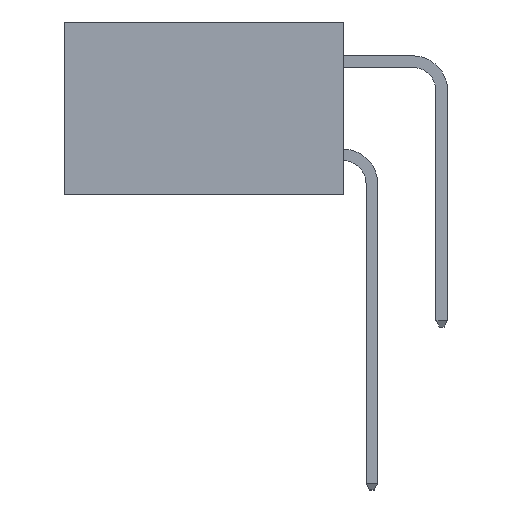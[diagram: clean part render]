
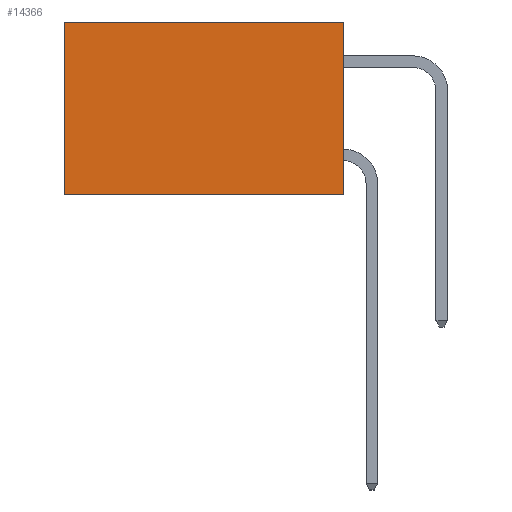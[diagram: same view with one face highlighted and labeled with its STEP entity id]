
A CAD part, left-side view. The second image highlights one B-rep face of the part: STEP entity #14366.
In plain terms, the highlighted planar face has unit normal (-1, 0, 0).
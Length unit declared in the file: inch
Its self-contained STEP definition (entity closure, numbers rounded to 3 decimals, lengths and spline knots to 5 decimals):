
#51 = VERTEX_POINT ( 'NONE', #115 ) ;
#115 = CARTESIAN_POINT ( 'NONE',  ( 0.2615, 0.6, 0. ) ) ;
#236 = PLANE ( 'NONE',  #11619 ) ;
#308 = CARTESIAN_POINT ( 'NONE',  ( 0.2615, 0., -0.37 ) ) ;
#563 = EDGE_CURVE ( 'NONE', #1393, #10285, #14573, .T. ) ;
#793 = CARTESIAN_POINT ( 'NONE',  ( 0.2615, 0., -0.37 ) ) ;
#1393 = VERTEX_POINT ( 'NONE', #1798 ) ;
#1501 = LINE ( 'NONE', #5867, #11359 ) ;
#1686 = VERTEX_POINT ( 'NONE', #12642 ) ;
#1798 = CARTESIAN_POINT ( 'NONE',  ( 0.2615, 0., 0. ) ) ;
#1828 = DIRECTION ( 'NONE',  ( 0., 0., -1. ) ) ;
#1860 = EDGE_CURVE ( 'NONE', #1393, #51, #1501, .T. ) ;
#4922 = VECTOR ( 'NONE', #1828, 39.37008 ) ;
#5165 = DIRECTION ( 'NONE',  ( 0., 1., 0. ) ) ;
#5459 = CARTESIAN_POINT ( 'NONE',  ( 0.2615, 0., -0.37 ) ) ;
#5867 = CARTESIAN_POINT ( 'NONE',  ( 0.2615, 0., 0. ) ) ;
#5938 = LINE ( 'NONE', #5459, #15102 ) ;
#6237 = DIRECTION ( 'NONE',  ( 0., 1., 0. ) ) ;
#6806 = LINE ( 'NONE', #13329, #15537 ) ;
#6842 = EDGE_LOOP ( 'NONE', ( #9838, #9909, #9921, #9937 ) ) ;
#6967 = FACE_OUTER_BOUND ( 'NONE', #6842, .T. ) ;
#9328 = DIRECTION ( 'NONE',  ( 0., 0., -1. ) ) ;
#9399 = DIRECTION ( 'NONE',  ( 1., 0., 0. ) ) ;
#9652 = EDGE_CURVE ( 'NONE', #10285, #1686, #5938, .T. ) ;
#9838 = ORIENTED_EDGE ( 'NONE', *, *, #13760, .T. ) ;
#9909 = ORIENTED_EDGE ( 'NONE', *, *, #9652, .F. ) ;
#9921 = ORIENTED_EDGE ( 'NONE', *, *, #563, .F. ) ;
#9937 = ORIENTED_EDGE ( 'NONE', *, *, #1860, .T. ) ;
#10285 = VERTEX_POINT ( 'NONE', #793 ) ;
#11359 = VECTOR ( 'NONE', #6237, 39.37008 ) ;
#11619 = AXIS2_PLACEMENT_3D ( 'NONE', #308, #9399, #9328 ) ;
#12350 = CARTESIAN_POINT ( 'NONE',  ( 0.2615, 0., -0.37 ) ) ;
#12642 = CARTESIAN_POINT ( 'NONE',  ( 0.2615, 0.6, -0.37 ) ) ;
#13218 = DIRECTION ( 'NONE',  ( 0., 0., -1. ) ) ;
#13329 = CARTESIAN_POINT ( 'NONE',  ( 0.2615, 0.6, -0.37 ) ) ;
#13760 = EDGE_CURVE ( 'NONE', #51, #1686, #6806, .T. ) ;
#14366 = ADVANCED_FACE ( 'NONE', ( #6967 ), #236, .F. ) ;
#14573 = LINE ( 'NONE', #12350, #4922 ) ;
#15102 = VECTOR ( 'NONE', #5165, 39.37008 ) ;
#15537 = VECTOR ( 'NONE', #13218, 39.37008 ) ;
